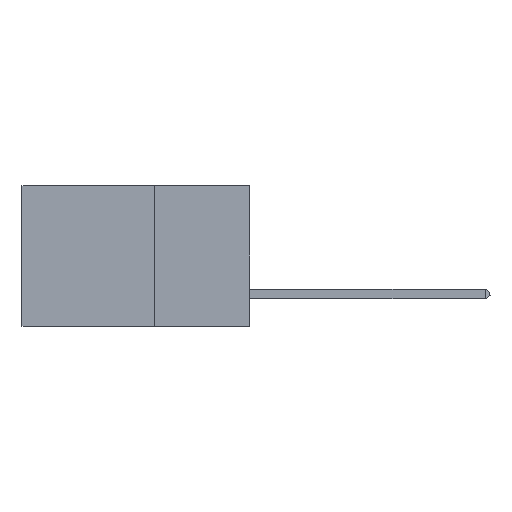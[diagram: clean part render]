
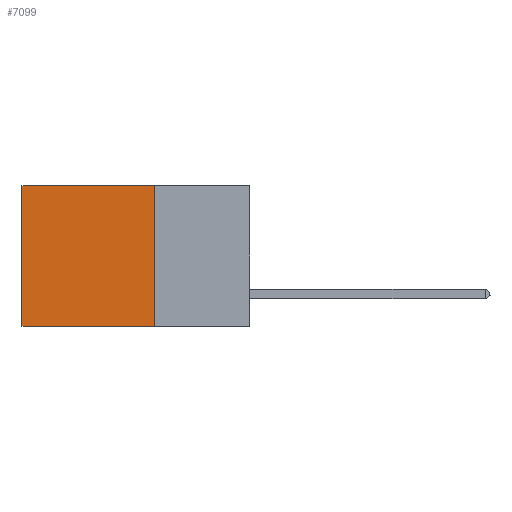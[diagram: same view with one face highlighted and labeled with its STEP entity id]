
A CAD part, left-side view. The second image highlights one B-rep face of the part: STEP entity #7099.
In plain terms, the highlighted planar face has unit normal (-1, 0, 0).
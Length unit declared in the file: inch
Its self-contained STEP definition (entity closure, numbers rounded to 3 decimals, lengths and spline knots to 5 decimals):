
#385 = DIRECTION ( 'NONE',  ( 0., 0., -1. ) ) ;
#691 = VERTEX_POINT ( 'NONE', #2352 ) ;
#735 = CARTESIAN_POINT ( 'NONE',  ( 0.2875, 0.25, -0.37 ) ) ;
#1068 = DIRECTION ( 'NONE',  ( 0., 0., -1. ) ) ;
#1080 = DIRECTION ( 'NONE',  ( 0., 1., 0. ) ) ;
#1299 = FACE_OUTER_BOUND ( 'NONE', #2734, .T. ) ;
#2088 = VECTOR ( 'NONE', #15026, 39.37008 ) ;
#2352 = CARTESIAN_POINT ( 'NONE',  ( 0.2875, 0.6, 0. ) ) ;
#2734 = EDGE_LOOP ( 'NONE', ( #13493, #10492, #10241, #7253 ) ) ;
#2982 = VECTOR ( 'NONE', #5264, 39.37008 ) ;
#3746 = LINE ( 'NONE', #10068, #2982 ) ;
#4613 = CARTESIAN_POINT ( 'NONE',  ( 0.2875, 0.25, 0. ) ) ;
#5063 = PLANE ( 'NONE',  #8415 ) ;
#5264 = DIRECTION ( 'NONE',  ( 0., 0., -1. ) ) ;
#5588 = VERTEX_POINT ( 'NONE', #12496 ) ;
#5849 = LINE ( 'NONE', #735, #2088 ) ;
#6596 = EDGE_CURVE ( 'NONE', #9890, #10044, #3746, .T. ) ;
#7099 = ADVANCED_FACE ( 'NONE', ( #1299 ), #5063, .F. ) ;
#7253 = ORIENTED_EDGE ( 'NONE', *, *, #10491, .T. ) ;
#7372 = EDGE_CURVE ( 'NONE', #691, #5588, #12668, .T. ) ;
#8415 = AXIS2_PLACEMENT_3D ( 'NONE', #9885, #11071, #385 ) ;
#9618 = LINE ( 'NONE', #4613, #12038 ) ;
#9885 = CARTESIAN_POINT ( 'NONE',  ( 0.2875, 0.25, 0. ) ) ;
#9890 = VERTEX_POINT ( 'NONE', #15236 ) ;
#10044 = VERTEX_POINT ( 'NONE', #13065 ) ;
#10068 = CARTESIAN_POINT ( 'NONE',  ( 0.2875, 0.25, 0. ) ) ;
#10241 = ORIENTED_EDGE ( 'NONE', *, *, #6596, .F. ) ;
#10491 = EDGE_CURVE ( 'NONE', #9890, #691, #9618, .T. ) ;
#10492 = ORIENTED_EDGE ( 'NONE', *, *, #12390, .F. ) ;
#10922 = CARTESIAN_POINT ( 'NONE',  ( 0.2875, 0.6, 0. ) ) ;
#11071 = DIRECTION ( 'NONE',  ( 1., 0., 0. ) ) ;
#12038 = VECTOR ( 'NONE', #1080, 39.37008 ) ;
#12390 = EDGE_CURVE ( 'NONE', #10044, #5588, #5849, .T. ) ;
#12496 = CARTESIAN_POINT ( 'NONE',  ( 0.2875, 0.6, -0.37 ) ) ;
#12668 = LINE ( 'NONE', #10922, #13984 ) ;
#13065 = CARTESIAN_POINT ( 'NONE',  ( 0.2875, 0.25, -0.37 ) ) ;
#13493 = ORIENTED_EDGE ( 'NONE', *, *, #7372, .T. ) ;
#13984 = VECTOR ( 'NONE', #1068, 39.37008 ) ;
#15026 = DIRECTION ( 'NONE',  ( 0., 1., 0. ) ) ;
#15236 = CARTESIAN_POINT ( 'NONE',  ( 0.2875, 0.25, 0. ) ) ;
